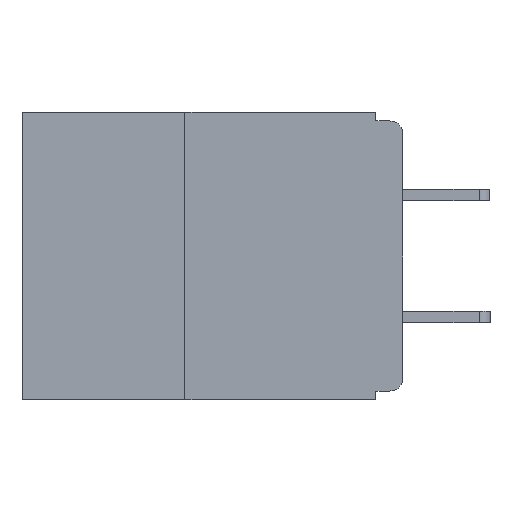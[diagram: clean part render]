
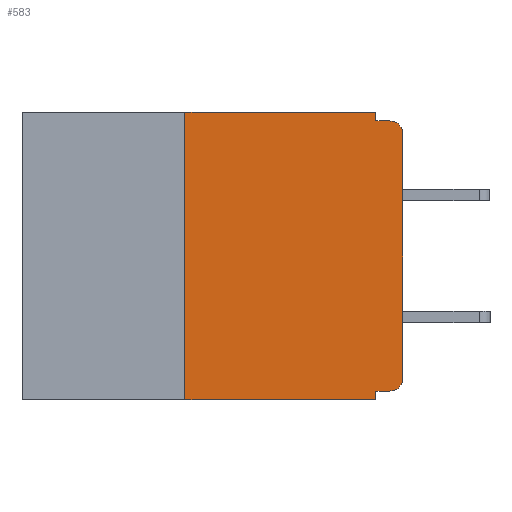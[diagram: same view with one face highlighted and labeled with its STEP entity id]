
A CAD part, left-side view. The second image highlights one B-rep face of the part: STEP entity #583.
In plain terms, the highlighted planar face has unit normal (-1, 0, 0).
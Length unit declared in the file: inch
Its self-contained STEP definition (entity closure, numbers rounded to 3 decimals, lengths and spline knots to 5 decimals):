
#583 = ADVANCED_FACE ( 'NONE', ( #16461 ), #20518, .F. ) ;
#693 = VERTEX_POINT ( 'NONE', #12473 ) ;
#896 = VECTOR ( 'NONE', #7386, 39.37008 ) ;
#1102 = VERTEX_POINT ( 'NONE', #3561 ) ;
#1274 = VERTEX_POINT ( 'NONE', #18329 ) ;
#1683 = EDGE_CURVE ( 'NONE', #19506, #1274, #17972, .T. ) ;
#1991 = ORIENTED_EDGE ( 'NONE', *, *, #13486, .T. ) ;
#2513 = LINE ( 'NONE', #7397, #18563 ) ;
#2759 = ORIENTED_EDGE ( 'NONE', *, *, #12524, .F. ) ;
#3561 = CARTESIAN_POINT ( 'NONE',  ( 0., 0., -0.025 ) ) ;
#4202 = CARTESIAN_POINT ( 'NONE',  ( 0., 0., -0.01 ) ) ;
#4631 = DIRECTION ( 'NONE',  ( 0., 1., 0. ) ) ;
#4645 = VERTEX_POINT ( 'NONE', #10032 ) ;
#4686 = CIRCLE ( 'NONE', #10031, 0.015 ) ;
#4910 = CARTESIAN_POINT ( 'NONE',  ( 0., 0.25, -0.33 ) ) ;
#5219 = AXIS2_PLACEMENT_3D ( 'NONE', #15051, #5424, #16644 ) ;
#5424 = DIRECTION ( 'NONE',  ( -1., 0., 0. ) ) ;
#5853 = VECTOR ( 'NONE', #15741, 39.37008 ) ;
#6228 = CARTESIAN_POINT ( 'NONE',  ( 0., 0.031, -0.33 ) ) ;
#6467 = DIRECTION ( 'NONE',  ( 0., 0., 1. ) ) ;
#6476 = VERTEX_POINT ( 'NONE', #6978 ) ;
#6726 = ORIENTED_EDGE ( 'NONE', *, *, #20761, .T. ) ;
#6853 = VERTEX_POINT ( 'NONE', #11094 ) ;
#6969 = ORIENTED_EDGE ( 'NONE', *, *, #19887, .F. ) ;
#6978 = CARTESIAN_POINT ( 'NONE',  ( 0., 0., -0.305 ) ) ;
#7381 = LINE ( 'NONE', #14139, #5853 ) ;
#7386 = DIRECTION ( 'NONE',  ( 0., -1., 0. ) ) ;
#7397 = CARTESIAN_POINT ( 'NONE',  ( 0., 0.437, -0.33 ) ) ;
#7586 = LINE ( 'NONE', #4910, #19417 ) ;
#7734 = ORIENTED_EDGE ( 'NONE', *, *, #17773, .T. ) ;
#7850 = CARTESIAN_POINT ( 'NONE',  ( 0., 0.015, -0.025 ) ) ;
#8074 = VECTOR ( 'NONE', #4631, 39.37008 ) ;
#8231 = LINE ( 'NONE', #15302, #11984 ) ;
#8561 = CARTESIAN_POINT ( 'NONE',  ( 0., 0.015, -0.32 ) ) ;
#8566 = DIRECTION ( 'NONE',  ( 0., 0., -1. ) ) ;
#8581 = EDGE_CURVE ( 'NONE', #6476, #1102, #8231, .T. ) ;
#8632 = CARTESIAN_POINT ( 'NONE',  ( 0., 0.031, -0.33 ) ) ;
#9204 = ORIENTED_EDGE ( 'NONE', *, *, #8581, .T. ) ;
#9334 = CARTESIAN_POINT ( 'NONE',  ( 0., 0., -0.32 ) ) ;
#9444 = DIRECTION ( 'NONE',  ( 0., 0., -1. ) ) ;
#10031 = AXIS2_PLACEMENT_3D ( 'NONE', #7850, #19107, #9444 ) ;
#10032 = CARTESIAN_POINT ( 'NONE',  ( 0., 0.031, 0. ) ) ;
#11035 = VERTEX_POINT ( 'NONE', #20642 ) ;
#11094 = CARTESIAN_POINT ( 'NONE',  ( 0., 0.25, -0.33 ) ) ;
#11796 = EDGE_CURVE ( 'NONE', #6853, #693, #7586, .T. ) ;
#11984 = VECTOR ( 'NONE', #18555, 39.37008 ) ;
#12199 = EDGE_CURVE ( 'NONE', #13106, #11035, #12336, .T. ) ;
#12336 = LINE ( 'NONE', #9334, #8074 ) ;
#12473 = CARTESIAN_POINT ( 'NONE',  ( 0., 0.25, 0. ) ) ;
#12524 = EDGE_CURVE ( 'NONE', #11035, #12835, #13746, .T. ) ;
#12588 = VECTOR ( 'NONE', #20757, 39.37008 ) ;
#12835 = VERTEX_POINT ( 'NONE', #6228 ) ;
#13025 = ORIENTED_EDGE ( 'NONE', *, *, #11796, .F. ) ;
#13083 = EDGE_LOOP ( 'NONE', ( #9204, #1991, #17806, #6969, #14303, #13025, #7734, #2759, #16035, #6726 ) ) ;
#13106 = VERTEX_POINT ( 'NONE', #8561 ) ;
#13485 = CARTESIAN_POINT ( 'NONE',  ( 0., 0.031, -0.01 ) ) ;
#13486 = EDGE_CURVE ( 'NONE', #1102, #1274, #4686, .T. ) ;
#13746 = LINE ( 'NONE', #8632, #17507 ) ;
#13874 = DIRECTION ( 'NONE',  ( 0., -1., 0. ) ) ;
#14139 = CARTESIAN_POINT ( 'NONE',  ( 0., 0.437, 0. ) ) ;
#14303 = ORIENTED_EDGE ( 'NONE', *, *, #14696, .F. ) ;
#14696 = EDGE_CURVE ( 'NONE', #693, #4645, #7381, .T. ) ;
#15051 = CARTESIAN_POINT ( 'NONE',  ( 0., 0.015, -0.305 ) ) ;
#15302 = CARTESIAN_POINT ( 'NONE',  ( 0., 0., 0. ) ) ;
#15741 = DIRECTION ( 'NONE',  ( 0., -1., 0. ) ) ;
#16035 = ORIENTED_EDGE ( 'NONE', *, *, #12199, .F. ) ;
#16461 = FACE_OUTER_BOUND ( 'NONE', #13083, .T. ) ;
#16644 = DIRECTION ( 'NONE',  ( 0., 0., -1. ) ) ;
#16849 = LINE ( 'NONE', #17609, #12588 ) ;
#17507 = VECTOR ( 'NONE', #8566, 39.37008 ) ;
#17609 = CARTESIAN_POINT ( 'NONE',  ( 0., 0.031, 0. ) ) ;
#17773 = EDGE_CURVE ( 'NONE', #6853, #12835, #2513, .T. ) ;
#17806 = ORIENTED_EDGE ( 'NONE', *, *, #1683, .F. ) ;
#17972 = LINE ( 'NONE', #4202, #896 ) ;
#17979 = DIRECTION ( 'NONE',  ( 1., 0., 0. ) ) ;
#18329 = CARTESIAN_POINT ( 'NONE',  ( 0., 0.015, -0.01 ) ) ;
#18555 = DIRECTION ( 'NONE',  ( 0., 0., 1. ) ) ;
#18563 = VECTOR ( 'NONE', #13874, 39.37008 ) ;
#18723 = AXIS2_PLACEMENT_3D ( 'NONE', #19535, #17979, #19697 ) ;
#19107 = DIRECTION ( 'NONE',  ( -1., 0., 0. ) ) ;
#19417 = VECTOR ( 'NONE', #6467, 39.37008 ) ;
#19506 = VERTEX_POINT ( 'NONE', #13485 ) ;
#19535 = CARTESIAN_POINT ( 'NONE',  ( 0., 0.437, 0. ) ) ;
#19697 = DIRECTION ( 'NONE',  ( 0., 0., -1. ) ) ;
#19887 = EDGE_CURVE ( 'NONE', #4645, #19506, #16849, .T. ) ;
#20518 = PLANE ( 'NONE',  #18723 ) ;
#20600 = CIRCLE ( 'NONE', #5219, 0.015 ) ;
#20642 = CARTESIAN_POINT ( 'NONE',  ( 0., 0.031, -0.32 ) ) ;
#20757 = DIRECTION ( 'NONE',  ( 0., 0., -1. ) ) ;
#20761 = EDGE_CURVE ( 'NONE', #13106, #6476, #20600, .T. ) ;
